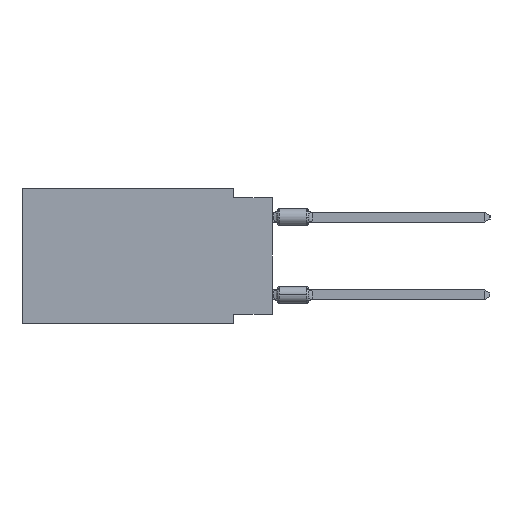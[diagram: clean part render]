
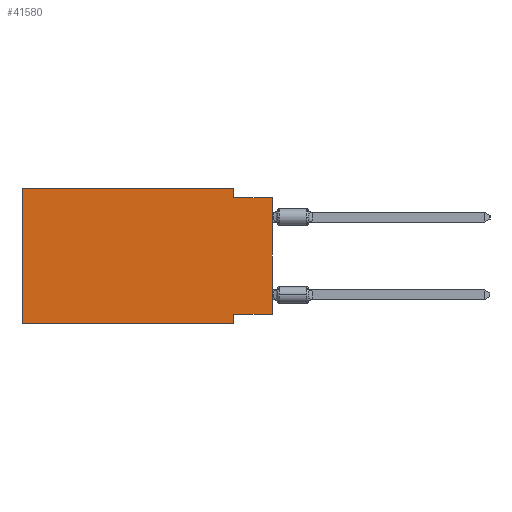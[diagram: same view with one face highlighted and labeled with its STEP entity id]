
A CAD part, left-side view. The second image highlights one B-rep face of the part: STEP entity #41580.
In plain terms, the highlighted planar face has unit normal (-1, 0, 0).
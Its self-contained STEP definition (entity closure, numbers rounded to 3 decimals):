
#838 = CARTESIAN_POINT ( 'NONE',  ( 0., 16.383, 0. ) ) ;
#1141 = ORIENTED_EDGE ( 'NONE', *, *, #35918, .T. ) ;
#1410 = CARTESIAN_POINT ( 'NONE',  ( 0., 2.54, -8.89 ) ) ;
#1668 = VERTEX_POINT ( 'NONE', #52725 ) ;
#2624 = DIRECTION ( 'NONE',  ( 0., 0., -1. ) ) ;
#3933 = VECTOR ( 'NONE', #33197, 1000. ) ;
#4876 = EDGE_CURVE ( 'NONE', #46525, #25403, #12634, .T. ) ;
#7797 = CARTESIAN_POINT ( 'NONE',  ( 0., 16.383, 0. ) ) ;
#8101 = CARTESIAN_POINT ( 'NONE',  ( 0., 0., -0.635 ) ) ;
#8411 = VECTOR ( 'NONE', #2624, 1000. ) ;
#9625 = ORIENTED_EDGE ( 'NONE', *, *, #32136, .F. ) ;
#10479 = DIRECTION ( 'NONE',  ( 0., -1., 0. ) ) ;
#11520 = VERTEX_POINT ( 'NONE', #23012 ) ;
#12634 = LINE ( 'NONE', #41909, #32054 ) ;
#12888 = EDGE_CURVE ( 'NONE', #18305, #1668, #61058, .T. ) ;
#14088 = DIRECTION ( 'NONE',  ( 0., -1., 0. ) ) ;
#14228 = ORIENTED_EDGE ( 'NONE', *, *, #46568, .T. ) ;
#14637 = CARTESIAN_POINT ( 'NONE',  ( 0., 2.54, -0.635 ) ) ;
#18204 = VERTEX_POINT ( 'NONE', #60137 ) ;
#18305 = VERTEX_POINT ( 'NONE', #32786 ) ;
#20072 = VECTOR ( 'NONE', #10479, 1000. ) ;
#21418 = CARTESIAN_POINT ( 'NONE',  ( 0., 0., -8.255 ) ) ;
#22021 = EDGE_LOOP ( 'NONE', ( #1141, #48835, #52162, #46225, #50043, #14228, #9625, #30303 ) ) ;
#23012 = CARTESIAN_POINT ( 'NONE',  ( 0., 0., -0.635 ) ) ;
#24336 = EDGE_CURVE ( 'NONE', #18204, #18305, #26908, .T. ) ;
#25403 = VERTEX_POINT ( 'NONE', #52339 ) ;
#25638 = EDGE_CURVE ( 'NONE', #39839, #11520, #53652, .T. ) ;
#26820 = DIRECTION ( 'NONE',  ( 0., 0., 1. ) ) ;
#26908 = LINE ( 'NONE', #53493, #3933 ) ;
#27900 = LINE ( 'NONE', #48183, #8411 ) ;
#30303 = ORIENTED_EDGE ( 'NONE', *, *, #4876, .F. ) ;
#30717 = VECTOR ( 'NONE', #26820, 1000. ) ;
#32054 = VECTOR ( 'NONE', #57547, 1000. ) ;
#32136 = EDGE_CURVE ( 'NONE', #25403, #41906, #39931, .T. ) ;
#32786 = CARTESIAN_POINT ( 'NONE',  ( 0., 16.383, 0. ) ) ;
#33197 = DIRECTION ( 'NONE',  ( 0., 0., 1. ) ) ;
#33275 = DIRECTION ( 'NONE',  ( 0., 0., -1. ) ) ;
#35584 = VECTOR ( 'NONE', #33275, 1000. ) ;
#35918 = EDGE_CURVE ( 'NONE', #46525, #11520, #45889, .T. ) ;
#38847 = VECTOR ( 'NONE', #42997, 1000. ) ;
#39839 = VERTEX_POINT ( 'NONE', #14637 ) ;
#39931 = LINE ( 'NONE', #44913, #35584 ) ;
#40693 = AXIS2_PLACEMENT_3D ( 'NONE', #7797, #53360, #43375 ) ;
#41580 = ADVANCED_FACE ( 'NONE', ( #64675 ), #53691, .F. ) ;
#41906 = VERTEX_POINT ( 'NONE', #1410 ) ;
#41909 = CARTESIAN_POINT ( 'NONE',  ( 0., 0., -8.255 ) ) ;
#42997 = DIRECTION ( 'NONE',  ( 0., -1., 0. ) ) ;
#43375 = DIRECTION ( 'NONE',  ( 0., 0., -1. ) ) ;
#44913 = CARTESIAN_POINT ( 'NONE',  ( 0., 2.54, -8.89 ) ) ;
#45889 = LINE ( 'NONE', #60557, #30717 ) ;
#46225 = ORIENTED_EDGE ( 'NONE', *, *, #12888, .F. ) ;
#46525 = VERTEX_POINT ( 'NONE', #21418 ) ;
#46568 = EDGE_CURVE ( 'NONE', #18204, #41906, #61994, .T. ) ;
#46684 = CARTESIAN_POINT ( 'NONE',  ( 0., 16.383, -8.89 ) ) ;
#48183 = CARTESIAN_POINT ( 'NONE',  ( 0., 2.54, 0. ) ) ;
#48835 = ORIENTED_EDGE ( 'NONE', *, *, #25638, .F. ) ;
#50043 = ORIENTED_EDGE ( 'NONE', *, *, #24336, .F. ) ;
#52162 = ORIENTED_EDGE ( 'NONE', *, *, #56287, .F. ) ;
#52339 = CARTESIAN_POINT ( 'NONE',  ( 0., 2.54, -8.255 ) ) ;
#52725 = CARTESIAN_POINT ( 'NONE',  ( 0., 2.54, 0. ) ) ;
#53360 = DIRECTION ( 'NONE',  ( 1., 0., 0. ) ) ;
#53493 = CARTESIAN_POINT ( 'NONE',  ( 0., 16.383, 0. ) ) ;
#53652 = LINE ( 'NONE', #8101, #54228 ) ;
#53691 = PLANE ( 'NONE',  #40693 ) ;
#54228 = VECTOR ( 'NONE', #14088, 1000. ) ;
#56287 = EDGE_CURVE ( 'NONE', #1668, #39839, #27900, .T. ) ;
#57547 = DIRECTION ( 'NONE',  ( 0., 1., 0. ) ) ;
#60137 = CARTESIAN_POINT ( 'NONE',  ( 0., 16.383, -8.89 ) ) ;
#60557 = CARTESIAN_POINT ( 'NONE',  ( 0., 0., 0. ) ) ;
#61058 = LINE ( 'NONE', #838, #20072 ) ;
#61994 = LINE ( 'NONE', #46684, #38847 ) ;
#64675 = FACE_OUTER_BOUND ( 'NONE', #22021, .T. ) ;
